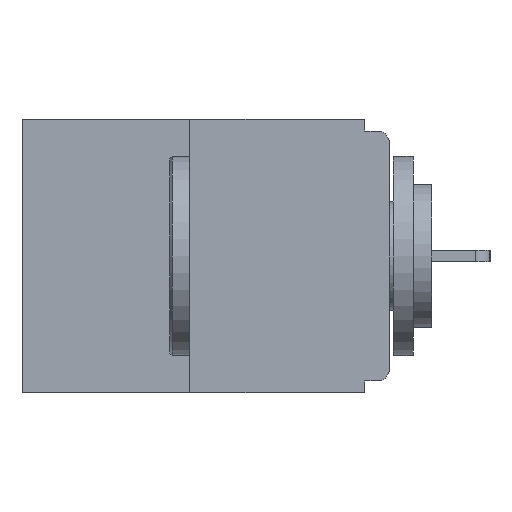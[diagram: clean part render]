
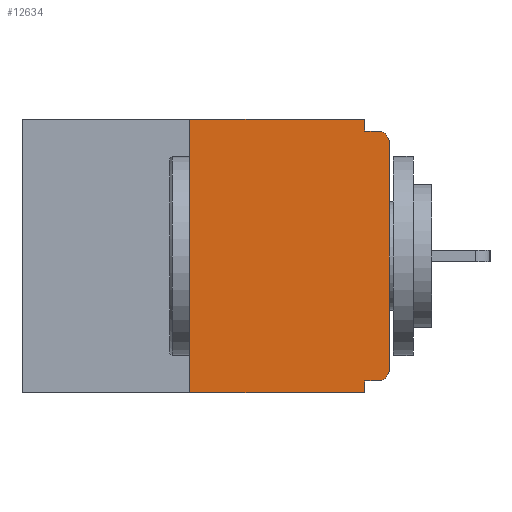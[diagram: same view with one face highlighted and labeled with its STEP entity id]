
A CAD part, left-side view. The second image highlights one B-rep face of the part: STEP entity #12634.
In plain terms, the highlighted planar face has unit normal (-1, 0, 0).
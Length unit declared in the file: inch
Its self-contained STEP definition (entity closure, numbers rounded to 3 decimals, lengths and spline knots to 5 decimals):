
#248 = AXIS2_PLACEMENT_3D ( 'NONE', #13043, #17193, #3687 ) ;
#432 = CARTESIAN_POINT ( 'NONE',  ( 0., 0.031, 0. ) ) ;
#1160 = LINE ( 'NONE', #11761, #15936 ) ;
#1465 = CARTESIAN_POINT ( 'NONE',  ( 0., 0.46, 0. ) ) ;
#1651 = CIRCLE ( 'NONE', #248, 0.015 ) ;
#2392 = EDGE_CURVE ( 'NONE', #10893, #4234, #9625, .T. ) ;
#2548 = CARTESIAN_POINT ( 'NONE',  ( 0., 0., 0. ) ) ;
#2551 = DIRECTION ( 'NONE',  ( 0., -1., 0. ) ) ;
#2795 = VERTEX_POINT ( 'NONE', #7717 ) ;
#3143 = FACE_OUTER_BOUND ( 'NONE', #18058, .T. ) ;
#3231 = EDGE_CURVE ( 'NONE', #9195, #22948, #1160, .T. ) ;
#3630 = CARTESIAN_POINT ( 'NONE',  ( 0., 0., -0.015 ) ) ;
#3687 = DIRECTION ( 'NONE',  ( 0., 0., -1. ) ) ;
#3874 = ORIENTED_EDGE ( 'NONE', *, *, #20666, .T. ) ;
#4234 = VERTEX_POINT ( 'NONE', #15056 ) ;
#4268 = CARTESIAN_POINT ( 'NONE',  ( 0., 0., -0.313 ) ) ;
#4313 = EDGE_CURVE ( 'NONE', #15343, #10346, #4376, .T. ) ;
#4376 = LINE ( 'NONE', #15551, #17050 ) ;
#4829 = CARTESIAN_POINT ( 'NONE',  ( 0., 0.031, -0.328 ) ) ;
#5131 = DIRECTION ( 'NONE',  ( 1., 0., 0. ) ) ;
#5491 = VECTOR ( 'NONE', #21704, 39.37008 ) ;
#5603 = LINE ( 'NONE', #21749, #14969 ) ;
#5821 = ORIENTED_EDGE ( 'NONE', *, *, #7571, .T. ) ;
#6939 = CIRCLE ( 'NONE', #13859, 0.015 ) ;
#7209 = ORIENTED_EDGE ( 'NONE', *, *, #4313, .F. ) ;
#7256 = LINE ( 'NONE', #3630, #13613 ) ;
#7571 = EDGE_CURVE ( 'NONE', #11950, #2795, #9129, .T. ) ;
#7717 = CARTESIAN_POINT ( 'NONE',  ( 0., 0., -0.03 ) ) ;
#7933 = DIRECTION ( 'NONE',  ( -1., 0., 0. ) ) ;
#8817 = EDGE_CURVE ( 'NONE', #22948, #10893, #5603, .T. ) ;
#9129 = LINE ( 'NONE', #2548, #22063 ) ;
#9195 = VERTEX_POINT ( 'NONE', #15174 ) ;
#9625 = LINE ( 'NONE', #432, #13557 ) ;
#9888 = DIRECTION ( 'NONE',  ( 0., 0., -1. ) ) ;
#10346 = VERTEX_POINT ( 'NONE', #4829 ) ;
#10893 = VERTEX_POINT ( 'NONE', #11553 ) ;
#11396 = ORIENTED_EDGE ( 'NONE', *, *, #3231, .F. ) ;
#11411 = DIRECTION ( 'NONE',  ( 0., 1., 0. ) ) ;
#11553 = CARTESIAN_POINT ( 'NONE',  ( 0., 0.031, 0. ) ) ;
#11675 = AXIS2_PLACEMENT_3D ( 'NONE', #1465, #5131, #16539 ) ;
#11761 = CARTESIAN_POINT ( 'NONE',  ( 0., 0.25, 0. ) ) ;
#11950 = VERTEX_POINT ( 'NONE', #4268 ) ;
#12292 = ORIENTED_EDGE ( 'NONE', *, *, #18500, .F. ) ;
#12293 = ORIENTED_EDGE ( 'NONE', *, *, #13820, .T. ) ;
#12380 = VECTOR ( 'NONE', #14155, 39.37008 ) ;
#12634 = ADVANCED_FACE ( 'NONE', ( #3143 ), #12967, .F. ) ;
#12967 = PLANE ( 'NONE',  #11675 ) ;
#13029 = LINE ( 'NONE', #14113, #5491 ) ;
#13043 = CARTESIAN_POINT ( 'NONE',  ( 0., 0.015, -0.313 ) ) ;
#13423 = ORIENTED_EDGE ( 'NONE', *, *, #2392, .F. ) ;
#13557 = VECTOR ( 'NONE', #17492, 39.37008 ) ;
#13613 = VECTOR ( 'NONE', #15037, 39.37008 ) ;
#13820 = EDGE_CURVE ( 'NONE', #9195, #14648, #13029, .T. ) ;
#13859 = AXIS2_PLACEMENT_3D ( 'NONE', #19484, #7933, #9888 ) ;
#14113 = CARTESIAN_POINT ( 'NONE',  ( 0., 0.46, -0.343 ) ) ;
#14155 = DIRECTION ( 'NONE',  ( 0., 0., -1. ) ) ;
#14223 = CARTESIAN_POINT ( 'NONE',  ( 0., 0.031, -0.343 ) ) ;
#14648 = VERTEX_POINT ( 'NONE', #16286 ) ;
#14780 = EDGE_CURVE ( 'NONE', #4234, #16740, #7256, .T. ) ;
#14969 = VECTOR ( 'NONE', #2551, 39.37008 ) ;
#15037 = DIRECTION ( 'NONE',  ( 0., -1., 0. ) ) ;
#15056 = CARTESIAN_POINT ( 'NONE',  ( 0., 0.031, -0.015 ) ) ;
#15123 = CARTESIAN_POINT ( 'NONE',  ( 0., 0.015, -0.328 ) ) ;
#15174 = CARTESIAN_POINT ( 'NONE',  ( 0., 0.25, -0.343 ) ) ;
#15343 = VERTEX_POINT ( 'NONE', #15123 ) ;
#15551 = CARTESIAN_POINT ( 'NONE',  ( 0., 0., -0.328 ) ) ;
#15936 = VECTOR ( 'NONE', #19604, 39.37008 ) ;
#16286 = CARTESIAN_POINT ( 'NONE',  ( 0., 0.031, -0.343 ) ) ;
#16539 = DIRECTION ( 'NONE',  ( 0., 0., -1. ) ) ;
#16740 = VERTEX_POINT ( 'NONE', #22922 ) ;
#17050 = VECTOR ( 'NONE', #11411, 39.37008 ) ;
#17193 = DIRECTION ( 'NONE',  ( -1., 0., 0. ) ) ;
#17492 = DIRECTION ( 'NONE',  ( 0., 0., -1. ) ) ;
#17730 = EDGE_CURVE ( 'NONE', #2795, #16740, #6939, .T. ) ;
#18058 = EDGE_LOOP ( 'NONE', ( #20948, #11396, #12293, #12292, #7209, #3874, #5821, #21911, #18949, #13423 ) ) ;
#18500 = EDGE_CURVE ( 'NONE', #10346, #14648, #20238, .T. ) ;
#18949 = ORIENTED_EDGE ( 'NONE', *, *, #14780, .F. ) ;
#19484 = CARTESIAN_POINT ( 'NONE',  ( 0., 0.015, -0.03 ) ) ;
#19604 = DIRECTION ( 'NONE',  ( 0., 0., 1. ) ) ;
#19639 = DIRECTION ( 'NONE',  ( 0., 0., 1. ) ) ;
#20238 = LINE ( 'NONE', #14223, #12380 ) ;
#20666 = EDGE_CURVE ( 'NONE', #15343, #11950, #1651, .T. ) ;
#20948 = ORIENTED_EDGE ( 'NONE', *, *, #8817, .F. ) ;
#21578 = CARTESIAN_POINT ( 'NONE',  ( 0., 0.25, 0. ) ) ;
#21704 = DIRECTION ( 'NONE',  ( 0., -1., 0. ) ) ;
#21749 = CARTESIAN_POINT ( 'NONE',  ( 0., 0.46, 0. ) ) ;
#21911 = ORIENTED_EDGE ( 'NONE', *, *, #17730, .T. ) ;
#22063 = VECTOR ( 'NONE', #19639, 39.37008 ) ;
#22922 = CARTESIAN_POINT ( 'NONE',  ( 0., 0.015, -0.015 ) ) ;
#22948 = VERTEX_POINT ( 'NONE', #21578 ) ;
